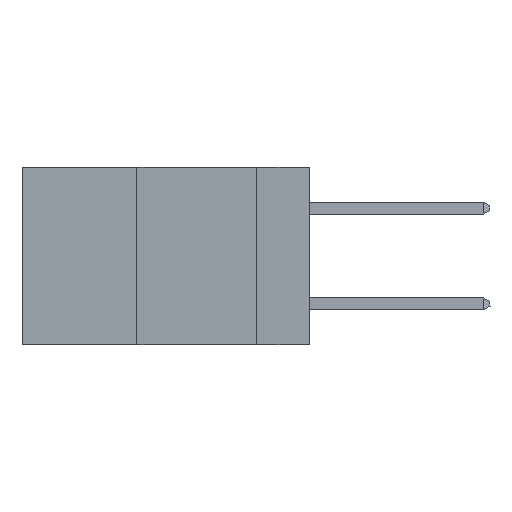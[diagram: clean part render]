
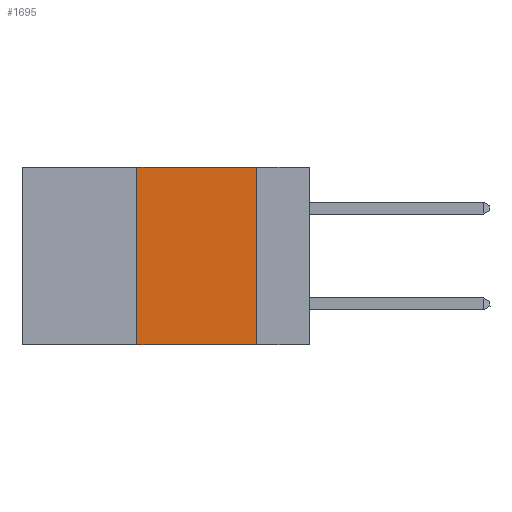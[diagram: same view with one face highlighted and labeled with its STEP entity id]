
A CAD part, left-side view. The second image highlights one B-rep face of the part: STEP entity #1695.
In plain terms, the highlighted planar face has unit normal (-1, 0, 0).
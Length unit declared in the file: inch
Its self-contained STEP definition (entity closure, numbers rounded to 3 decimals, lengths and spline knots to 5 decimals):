
#551 = LINE ( 'NONE', #5291, #9588 ) ;
#985 = ORIENTED_EDGE ( 'NONE', *, *, #16023, .F. ) ;
#1258 = CARTESIAN_POINT ( 'NONE',  ( 0., 0.11, 0. ) ) ;
#1566 = CARTESIAN_POINT ( 'NONE',  ( 0., 0.11, -0.37 ) ) ;
#1645 = CARTESIAN_POINT ( 'NONE',  ( 0., 0.36, 0. ) ) ;
#1695 = ADVANCED_FACE ( 'NONE', ( #3879 ), #17941, .F. ) ;
#2828 = LINE ( 'NONE', #1645, #15817 ) ;
#3170 = DIRECTION ( 'NONE',  ( 0., 0., -1. ) ) ;
#3531 = DIRECTION ( 'NONE',  ( 0., 0., 1. ) ) ;
#3879 = FACE_OUTER_BOUND ( 'NONE', #6992, .T. ) ;
#5291 = CARTESIAN_POINT ( 'NONE',  ( 0., 0.6, -0.37 ) ) ;
#6878 = VERTEX_POINT ( 'NONE', #15188 ) ;
#6992 = EDGE_LOOP ( 'NONE', ( #985, #11059, #16868, #22753 ) ) ;
#7061 = DIRECTION ( 'NONE',  ( 0., -1., 0. ) ) ;
#8255 = EDGE_CURVE ( 'NONE', #8755, #16619, #551, .T. ) ;
#8755 = VERTEX_POINT ( 'NONE', #15350 ) ;
#9184 = DIRECTION ( 'NONE',  ( 1., 0., 0. ) ) ;
#9435 = EDGE_CURVE ( 'NONE', #8755, #14977, #2828, .T. ) ;
#9588 = VECTOR ( 'NONE', #7061, 39.37008 ) ;
#11059 = ORIENTED_EDGE ( 'NONE', *, *, #15454, .F. ) ;
#12336 = AXIS2_PLACEMENT_3D ( 'NONE', #21458, #9184, #21535 ) ;
#12807 = VECTOR ( 'NONE', #3170, 39.37008 ) ;
#14977 = VERTEX_POINT ( 'NONE', #18035 ) ;
#15188 = CARTESIAN_POINT ( 'NONE',  ( 0., 0.11, 0. ) ) ;
#15350 = CARTESIAN_POINT ( 'NONE',  ( 0., 0.36, -0.37 ) ) ;
#15454 = EDGE_CURVE ( 'NONE', #14977, #6878, #18438, .T. ) ;
#15817 = VECTOR ( 'NONE', #3531, 39.37008 ) ;
#16023 = EDGE_CURVE ( 'NONE', #6878, #16619, #19766, .T. ) ;
#16619 = VERTEX_POINT ( 'NONE', #1566 ) ;
#16868 = ORIENTED_EDGE ( 'NONE', *, *, #9435, .F. ) ;
#17482 = DIRECTION ( 'NONE',  ( 0., -1., 0. ) ) ;
#17868 = VECTOR ( 'NONE', #17482, 39.37008 ) ;
#17941 = PLANE ( 'NONE',  #12336 ) ;
#18035 = CARTESIAN_POINT ( 'NONE',  ( 0., 0.36, 0. ) ) ;
#18438 = LINE ( 'NONE', #20980, #17868 ) ;
#19766 = LINE ( 'NONE', #1258, #12807 ) ;
#20980 = CARTESIAN_POINT ( 'NONE',  ( 0., 0.6, 0. ) ) ;
#21458 = CARTESIAN_POINT ( 'NONE',  ( 0., 0.6, 0. ) ) ;
#21535 = DIRECTION ( 'NONE',  ( 0., 0., -1. ) ) ;
#22753 = ORIENTED_EDGE ( 'NONE', *, *, #8255, .T. ) ;
